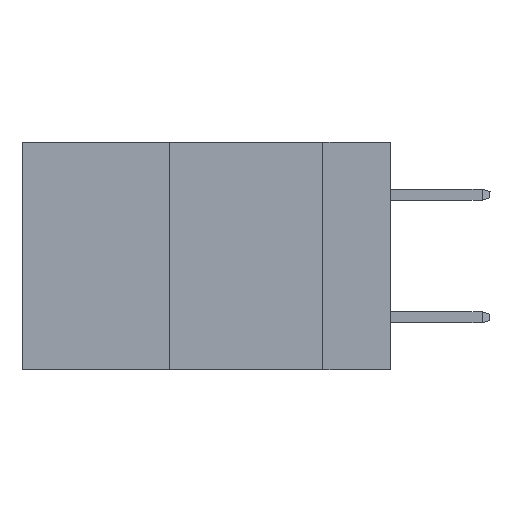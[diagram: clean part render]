
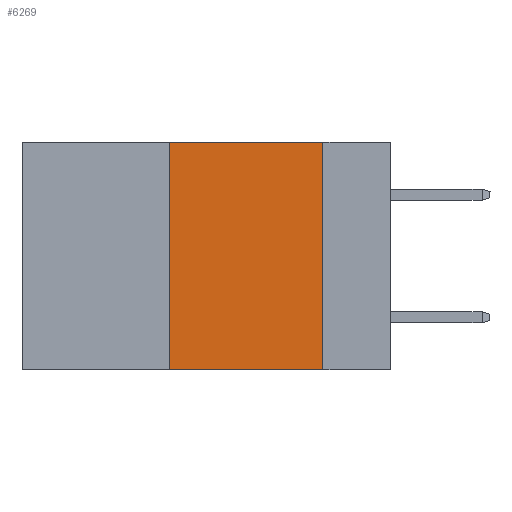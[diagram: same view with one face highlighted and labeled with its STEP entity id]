
A CAD part, left-side view. The second image highlights one B-rep face of the part: STEP entity #6269.
In plain terms, the highlighted planar face has unit normal (-1, 0, 0).
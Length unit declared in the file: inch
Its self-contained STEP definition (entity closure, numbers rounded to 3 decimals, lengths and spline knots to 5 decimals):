
#363 = VECTOR ( 'NONE', #950, 39.37008 ) ;
#507 = ORIENTED_EDGE ( 'NONE', *, *, #3722, .F. ) ;
#702 = FACE_OUTER_BOUND ( 'NONE', #1473, .T. ) ;
#757 = ORIENTED_EDGE ( 'NONE', *, *, #2086, .F. ) ;
#940 = VECTOR ( 'NONE', #6389, 39.37008 ) ;
#950 = DIRECTION ( 'NONE',  ( 0., 0., -1. ) ) ;
#1001 = ORIENTED_EDGE ( 'NONE', *, *, #4716, .F. ) ;
#1332 = DIRECTION ( 'NONE',  ( 0., -1., 0. ) ) ;
#1422 = CARTESIAN_POINT ( 'NONE',  ( 0., 0.6, -0.37 ) ) ;
#1473 = EDGE_LOOP ( 'NONE', ( #507, #1001, #757, #3479 ) ) ;
#1745 = CARTESIAN_POINT ( 'NONE',  ( 0., 0.11, -0.37 ) ) ;
#2086 = EDGE_CURVE ( 'NONE', #4125, #5802, #8168, .T. ) ;
#2200 = CARTESIAN_POINT ( 'NONE',  ( 0., 0.11, 0. ) ) ;
#2487 = VERTEX_POINT ( 'NONE', #4074 ) ;
#2615 = CARTESIAN_POINT ( 'NONE',  ( 0., 0.6, 0. ) ) ;
#2796 = LINE ( 'NONE', #8465, #4376 ) ;
#3440 = CARTESIAN_POINT ( 'NONE',  ( 0., 0.36, 0. ) ) ;
#3479 = ORIENTED_EDGE ( 'NONE', *, *, #4741, .T. ) ;
#3722 = EDGE_CURVE ( 'NONE', #2487, #7320, #8248, .T. ) ;
#3980 = CARTESIAN_POINT ( 'NONE',  ( 0., 0.36, 0. ) ) ;
#4074 = CARTESIAN_POINT ( 'NONE',  ( 0., 0.11, 0. ) ) ;
#4125 = VERTEX_POINT ( 'NONE', #5667 ) ;
#4376 = VECTOR ( 'NONE', #1332, 39.37008 ) ;
#4620 = AXIS2_PLACEMENT_3D ( 'NONE', #2615, #8204, #5603 ) ;
#4716 = EDGE_CURVE ( 'NONE', #5802, #2487, #2796, .T. ) ;
#4741 = EDGE_CURVE ( 'NONE', #4125, #7320, #5932, .T. ) ;
#5603 = DIRECTION ( 'NONE',  ( 0., 0., -1. ) ) ;
#5667 = CARTESIAN_POINT ( 'NONE',  ( 0., 0.36, -0.37 ) ) ;
#5802 = VERTEX_POINT ( 'NONE', #3980 ) ;
#5932 = LINE ( 'NONE', #1422, #940 ) ;
#6269 = ADVANCED_FACE ( 'NONE', ( #702 ), #8234, .F. ) ;
#6389 = DIRECTION ( 'NONE',  ( 0., -1., 0. ) ) ;
#7320 = VERTEX_POINT ( 'NONE', #1745 ) ;
#7731 = VECTOR ( 'NONE', #8411, 39.37008 ) ;
#8168 = LINE ( 'NONE', #3440, #7731 ) ;
#8204 = DIRECTION ( 'NONE',  ( 1., 0., 0. ) ) ;
#8234 = PLANE ( 'NONE',  #4620 ) ;
#8248 = LINE ( 'NONE', #2200, #363 ) ;
#8411 = DIRECTION ( 'NONE',  ( 0., 0., 1. ) ) ;
#8465 = CARTESIAN_POINT ( 'NONE',  ( 0., 0.6, 0. ) ) ;
